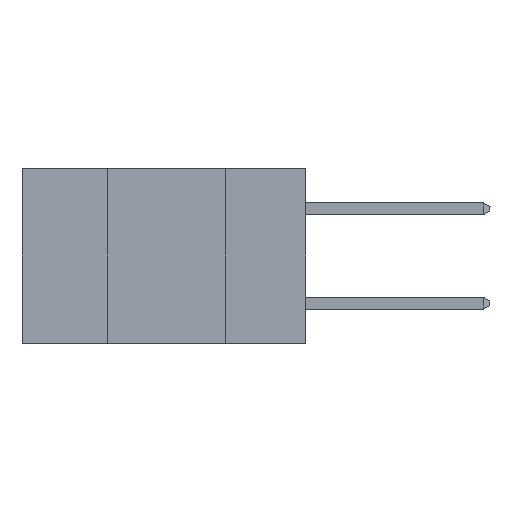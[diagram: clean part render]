
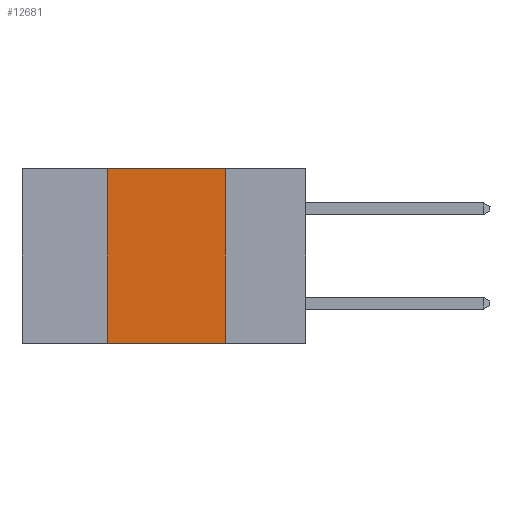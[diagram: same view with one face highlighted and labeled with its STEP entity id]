
A CAD part, left-side view. The second image highlights one B-rep face of the part: STEP entity #12681.
In plain terms, the highlighted planar face has unit normal (-1, 0, 0).
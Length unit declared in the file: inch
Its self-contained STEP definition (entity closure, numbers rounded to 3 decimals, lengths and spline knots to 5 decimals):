
#256 = EDGE_LOOP ( 'NONE', ( #22639, #15751, #18119, #7833 ) ) ;
#771 = DIRECTION ( 'NONE',  ( 0., 0., -1. ) ) ;
#2378 = CARTESIAN_POINT ( 'NONE',  ( 0., 0.6, -0.37 ) ) ;
#3241 = VECTOR ( 'NONE', #13599, 39.37008 ) ;
#4097 = LINE ( 'NONE', #11789, #3241 ) ;
#4435 = CARTESIAN_POINT ( 'NONE',  ( 0., 0.42, -0.37 ) ) ;
#5567 = DIRECTION ( 'NONE',  ( 0., 0., -1. ) ) ;
#6097 = CARTESIAN_POINT ( 'NONE',  ( 0., 0.6, 0. ) ) ;
#6187 = VERTEX_POINT ( 'NONE', #21968 ) ;
#6294 = EDGE_CURVE ( 'NONE', #12670, #6996, #4097, .T. ) ;
#6996 = VERTEX_POINT ( 'NONE', #16885 ) ;
#7062 = AXIS2_PLACEMENT_3D ( 'NONE', #15493, #15744, #771 ) ;
#7833 = ORIENTED_EDGE ( 'NONE', *, *, #12921, .T. ) ;
#8617 = VERTEX_POINT ( 'NONE', #23492 ) ;
#9097 = LINE ( 'NONE', #6097, #14080 ) ;
#10772 = VECTOR ( 'NONE', #15550, 39.37008 ) ;
#11566 = EDGE_CURVE ( 'NONE', #6996, #8617, #9097, .T. ) ;
#11640 = LINE ( 'NONE', #13007, #18122 ) ;
#11789 = CARTESIAN_POINT ( 'NONE',  ( 0., 0.42, 0. ) ) ;
#12670 = VERTEX_POINT ( 'NONE', #4435 ) ;
#12681 = ADVANCED_FACE ( 'NONE', ( #21055 ), #23089, .F. ) ;
#12921 = EDGE_CURVE ( 'NONE', #12670, #6187, #16038, .T. ) ;
#13007 = CARTESIAN_POINT ( 'NONE',  ( 0., 0.17, 0. ) ) ;
#13599 = DIRECTION ( 'NONE',  ( 0., 0., 1. ) ) ;
#14080 = VECTOR ( 'NONE', #15462, 39.37008 ) ;
#15462 = DIRECTION ( 'NONE',  ( 0., -1., 0. ) ) ;
#15493 = CARTESIAN_POINT ( 'NONE',  ( 0., 0.6, 0. ) ) ;
#15550 = DIRECTION ( 'NONE',  ( 0., -1., 0. ) ) ;
#15744 = DIRECTION ( 'NONE',  ( 1., 0., 0. ) ) ;
#15751 = ORIENTED_EDGE ( 'NONE', *, *, #11566, .F. ) ;
#16038 = LINE ( 'NONE', #2378, #10772 ) ;
#16885 = CARTESIAN_POINT ( 'NONE',  ( 0., 0.42, 0. ) ) ;
#17311 = EDGE_CURVE ( 'NONE', #8617, #6187, #11640, .T. ) ;
#18119 = ORIENTED_EDGE ( 'NONE', *, *, #6294, .F. ) ;
#18122 = VECTOR ( 'NONE', #5567, 39.37008 ) ;
#21055 = FACE_OUTER_BOUND ( 'NONE', #256, .T. ) ;
#21968 = CARTESIAN_POINT ( 'NONE',  ( 0., 0.17, -0.37 ) ) ;
#22639 = ORIENTED_EDGE ( 'NONE', *, *, #17311, .F. ) ;
#23089 = PLANE ( 'NONE',  #7062 ) ;
#23492 = CARTESIAN_POINT ( 'NONE',  ( 0., 0.17, 0. ) ) ;
